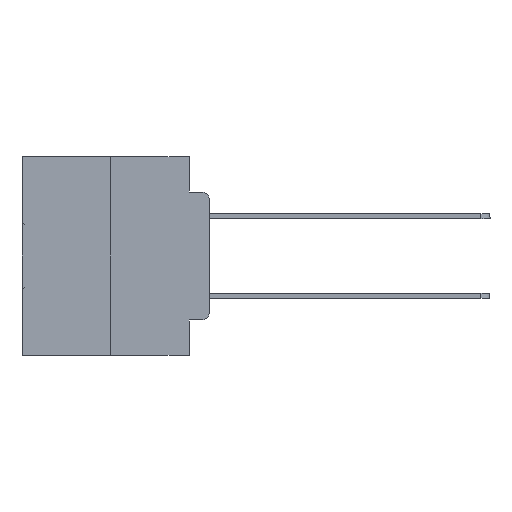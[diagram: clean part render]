
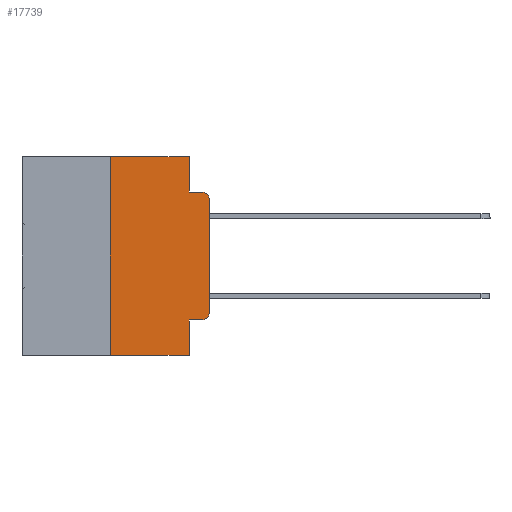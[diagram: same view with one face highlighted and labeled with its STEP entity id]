
A CAD part, left-side view. The second image highlights one B-rep face of the part: STEP entity #17739.
In plain terms, the highlighted planar face has unit normal (-1, 0, 0).
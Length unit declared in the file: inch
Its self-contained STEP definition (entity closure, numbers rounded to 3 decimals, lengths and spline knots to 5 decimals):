
#25 = VECTOR ( 'NONE', #31363, 39.37008 ) ;
#240 = VERTEX_POINT ( 'NONE', #17389 ) ;
#619 = CARTESIAN_POINT ( 'NONE',  ( 0., 0.473, 0. ) ) ;
#734 = PLANE ( 'NONE',  #13747 ) ;
#841 = LINE ( 'NONE', #19229, #25 ) ;
#983 = VERTEX_POINT ( 'NONE', #9730 ) ;
#1161 = EDGE_CURVE ( 'NONE', #24898, #16958, #10043, .T. ) ;
#1270 = VECTOR ( 'NONE', #17307, 39.37008 ) ;
#1729 = ORIENTED_EDGE ( 'NONE', *, *, #19271, .T. ) ;
#2756 = VECTOR ( 'NONE', #17810, 39.37008 ) ;
#2896 = EDGE_CURVE ( 'NONE', #9101, #26798, #841, .T. ) ;
#3100 = CARTESIAN_POINT ( 'NONE',  ( 0., 0.051, 0. ) ) ;
#3308 = CARTESIAN_POINT ( 'NONE',  ( 0., 0.051, -0.4115 ) ) ;
#3310 = CARTESIAN_POINT ( 'NONE',  ( 0., 0.25, -0.5 ) ) ;
#3317 = DIRECTION ( 'NONE',  ( 0., 0., -1. ) ) ;
#3601 = CARTESIAN_POINT ( 'NONE',  ( 0., 0.25, 0. ) ) ;
#4120 = ORIENTED_EDGE ( 'NONE', *, *, #2896, .F. ) ;
#4486 = CARTESIAN_POINT ( 'NONE',  ( 0., 0.051, 0. ) ) ;
#4888 = VECTOR ( 'NONE', #7892, 39.37008 ) ;
#4926 = ORIENTED_EDGE ( 'NONE', *, *, #1161, .F. ) ;
#5377 = CARTESIAN_POINT ( 'NONE',  ( 0., 0.051, -0.4115 ) ) ;
#6875 = ORIENTED_EDGE ( 'NONE', *, *, #28977, .T. ) ;
#7190 = DIRECTION ( 'NONE',  ( 0., 0., -1. ) ) ;
#7892 = DIRECTION ( 'NONE',  ( 0., -1., 0. ) ) ;
#8910 = VERTEX_POINT ( 'NONE', #27256 ) ;
#9101 = VERTEX_POINT ( 'NONE', #3310 ) ;
#9659 = LINE ( 'NONE', #4486, #16991 ) ;
#9730 = CARTESIAN_POINT ( 'NONE',  ( 0., 0.051, -0.0885 ) ) ;
#10043 = LINE ( 'NONE', #3100, #16550 ) ;
#10218 = CARTESIAN_POINT ( 'NONE',  ( 0., 0.051, -0.5 ) ) ;
#10237 = DIRECTION ( 'NONE',  ( -1., 0., 0. ) ) ;
#11317 = EDGE_CURVE ( 'NONE', #28053, #983, #9659, .T. ) ;
#11727 = CARTESIAN_POINT ( 'NONE',  ( 0., 0.02, -0.3915 ) ) ;
#12353 = CARTESIAN_POINT ( 'NONE',  ( 0., 0.473, 0. ) ) ;
#12475 = EDGE_CURVE ( 'NONE', #9101, #16958, #14995, .T. ) ;
#13128 = ORIENTED_EDGE ( 'NONE', *, *, #25083, .T. ) ;
#13747 = AXIS2_PLACEMENT_3D ( 'NONE', #619, #18237, #3317 ) ;
#14176 = DIRECTION ( 'NONE',  ( 0., 0., -1. ) ) ;
#14609 = LINE ( 'NONE', #12353, #1270 ) ;
#14995 = LINE ( 'NONE', #29126, #27195 ) ;
#15043 = ORIENTED_EDGE ( 'NONE', *, *, #17605, .F. ) ;
#15202 = CIRCLE ( 'NONE', #17321, 0.02 ) ;
#16550 = VECTOR ( 'NONE', #7190, 39.37008 ) ;
#16553 = ORIENTED_EDGE ( 'NONE', *, *, #22207, .F. ) ;
#16958 = VERTEX_POINT ( 'NONE', #10218 ) ;
#16991 = VECTOR ( 'NONE', #19371, 39.37008 ) ;
#17085 = CARTESIAN_POINT ( 'NONE',  ( 0., 0., -0.3915 ) ) ;
#17168 = VERTEX_POINT ( 'NONE', #30534 ) ;
#17307 = DIRECTION ( 'NONE',  ( 0., -1., 0. ) ) ;
#17321 = AXIS2_PLACEMENT_3D ( 'NONE', #24940, #10237, #27322 ) ;
#17333 = LINE ( 'NONE', #5377, #4888 ) ;
#17389 = CARTESIAN_POINT ( 'NONE',  ( 0., 0.02, -0.0885 ) ) ;
#17543 = LINE ( 'NONE', #18737, #31188 ) ;
#17605 = EDGE_CURVE ( 'NONE', #983, #240, #28949, .T. ) ;
#17739 = ADVANCED_FACE ( 'NONE', ( #31578 ), #734, .F. ) ;
#17810 = DIRECTION ( 'NONE',  ( 0., -1., 0. ) ) ;
#18237 = DIRECTION ( 'NONE',  ( 1., 0., 0. ) ) ;
#18737 = CARTESIAN_POINT ( 'NONE',  ( 0., 0., 0. ) ) ;
#19229 = CARTESIAN_POINT ( 'NONE',  ( 0., 0.25, 0. ) ) ;
#19271 = EDGE_CURVE ( 'NONE', #8910, #240, #15202, .T. ) ;
#19316 = AXIS2_PLACEMENT_3D ( 'NONE', #11727, #28770, #14176 ) ;
#19371 = DIRECTION ( 'NONE',  ( 0., 0., -1. ) ) ;
#19520 = DIRECTION ( 'NONE',  ( 0., -1., 0. ) ) ;
#21212 = DIRECTION ( 'NONE',  ( 0., 0., 1. ) ) ;
#22207 = EDGE_CURVE ( 'NONE', #26798, #28053, #14609, .T. ) ;
#24033 = VERTEX_POINT ( 'NONE', #17085 ) ;
#24898 = VERTEX_POINT ( 'NONE', #3308 ) ;
#24940 = CARTESIAN_POINT ( 'NONE',  ( 0., 0.02, -0.1085 ) ) ;
#25066 = CARTESIAN_POINT ( 'NONE',  ( 0., 0.051, -0.0885 ) ) ;
#25083 = EDGE_CURVE ( 'NONE', #17168, #24033, #31024, .T. ) ;
#25375 = ORIENTED_EDGE ( 'NONE', *, *, #31503, .T. ) ;
#26798 = VERTEX_POINT ( 'NONE', #3601 ) ;
#27195 = VECTOR ( 'NONE', #19520, 39.37008 ) ;
#27256 = CARTESIAN_POINT ( 'NONE',  ( 0., 0., -0.1085 ) ) ;
#27322 = DIRECTION ( 'NONE',  ( 0., 0., -1. ) ) ;
#28053 = VERTEX_POINT ( 'NONE', #29491 ) ;
#28730 = ORIENTED_EDGE ( 'NONE', *, *, #11317, .F. ) ;
#28770 = DIRECTION ( 'NONE',  ( -1., 0., 0. ) ) ;
#28949 = LINE ( 'NONE', #25066, #2756 ) ;
#28977 = EDGE_CURVE ( 'NONE', #24033, #8910, #17543, .T. ) ;
#29126 = CARTESIAN_POINT ( 'NONE',  ( 0., 0.473, -0.5 ) ) ;
#29491 = CARTESIAN_POINT ( 'NONE',  ( 0., 0.051, 0. ) ) ;
#30246 = ORIENTED_EDGE ( 'NONE', *, *, #12475, .T. ) ;
#30534 = CARTESIAN_POINT ( 'NONE',  ( 0., 0.02, -0.4115 ) ) ;
#31024 = CIRCLE ( 'NONE', #19316, 0.02 ) ;
#31188 = VECTOR ( 'NONE', #21212, 39.37008 ) ;
#31363 = DIRECTION ( 'NONE',  ( 0., 0., 1. ) ) ;
#31503 = EDGE_CURVE ( 'NONE', #24898, #17168, #17333, .T. ) ;
#31578 = FACE_OUTER_BOUND ( 'NONE', #31666, .T. ) ;
#31666 = EDGE_LOOP ( 'NONE', ( #6875, #1729, #15043, #28730, #16553, #4120, #30246, #4926, #25375, #13128 ) ) ;
